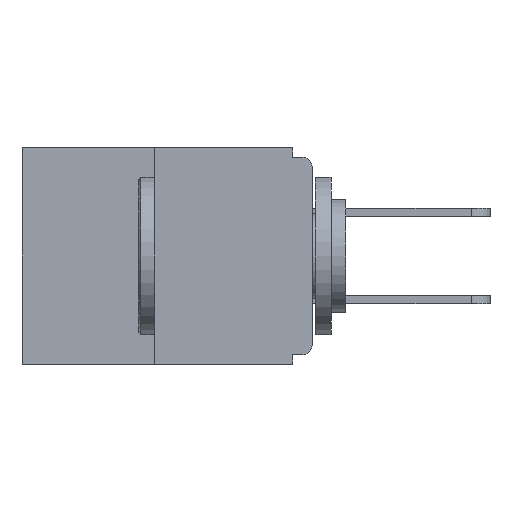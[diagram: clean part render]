
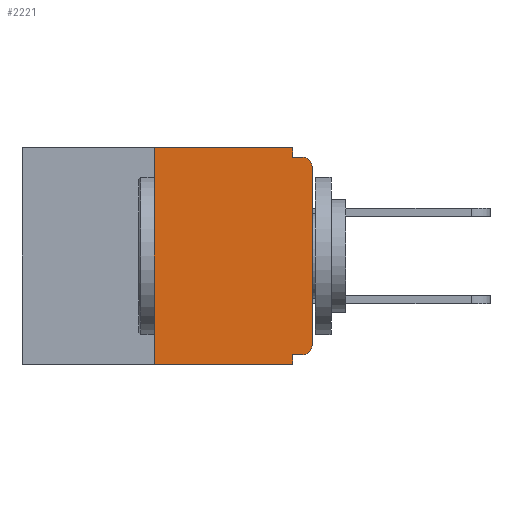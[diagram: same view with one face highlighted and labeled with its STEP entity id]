
A CAD part, left-side view. The second image highlights one B-rep face of the part: STEP entity #2221.
In plain terms, the highlighted planar face has unit normal (-1, 0, 0).
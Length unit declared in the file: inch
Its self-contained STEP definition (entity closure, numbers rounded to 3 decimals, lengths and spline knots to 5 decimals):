
#11 = CARTESIAN_POINT ( 'NONE',  ( 0., 0.031, -0.015 ) ) ;
#35 = DIRECTION ( 'NONE',  ( 1., 0., 0. ) ) ;
#146 = CARTESIAN_POINT ( 'NONE',  ( 0., 0., -0.328 ) ) ;
#283 = EDGE_CURVE ( 'NONE', #6004, #7386, #11529, .T. ) ;
#338 = CARTESIAN_POINT ( 'NONE',  ( 0., 0.031, 0. ) ) ;
#627 = AXIS2_PLACEMENT_3D ( 'NONE', #953, #35, #7451 ) ;
#688 = EDGE_CURVE ( 'NONE', #5996, #1993, #7983, .T. ) ;
#821 = DIRECTION ( 'NONE',  ( 0., 0., 1. ) ) ;
#953 = CARTESIAN_POINT ( 'NONE',  ( 0., 0.46, 0. ) ) ;
#961 = ORIENTED_EDGE ( 'NONE', *, *, #6815, .F. ) ;
#1276 = LINE ( 'NONE', #10023, #9420 ) ;
#1519 = VERTEX_POINT ( 'NONE', #7394 ) ;
#1734 = EDGE_CURVE ( 'NONE', #5830, #1993, #1919, .T. ) ;
#1814 = ORIENTED_EDGE ( 'NONE', *, *, #283, .F. ) ;
#1919 = LINE ( 'NONE', #5039, #4469 ) ;
#1963 = VERTEX_POINT ( 'NONE', #5065 ) ;
#1993 = VERTEX_POINT ( 'NONE', #6991 ) ;
#2065 = CARTESIAN_POINT ( 'NONE',  ( 0., 0., -0.03 ) ) ;
#2221 = ADVANCED_FACE ( 'NONE', ( #7251 ), #2738, .F. ) ;
#2358 = DIRECTION ( 'NONE',  ( 0., -1., 0. ) ) ;
#2637 = CARTESIAN_POINT ( 'NONE',  ( 0., 0.031, -0.343 ) ) ;
#2713 = VECTOR ( 'NONE', #10312, 39.37008 ) ;
#2722 = VERTEX_POINT ( 'NONE', #8371 ) ;
#2738 = PLANE ( 'NONE',  #627 ) ;
#2807 = DIRECTION ( 'NONE',  ( -1., 0., 0. ) ) ;
#2869 = DIRECTION ( 'NONE',  ( 0., 0., -1. ) ) ;
#2889 = CARTESIAN_POINT ( 'NONE',  ( 0., 0.25, 0. ) ) ;
#2900 = CARTESIAN_POINT ( 'NONE',  ( 0., 0.015, -0.03 ) ) ;
#3230 = EDGE_CURVE ( 'NONE', #7386, #5830, #5645, .T. ) ;
#3302 = EDGE_CURVE ( 'NONE', #11830, #5996, #1276, .T. ) ;
#3470 = LINE ( 'NONE', #2637, #6813 ) ;
#3475 = ORIENTED_EDGE ( 'NONE', *, *, #1734, .F. ) ;
#3624 = AXIS2_PLACEMENT_3D ( 'NONE', #4857, #5897, #11465 ) ;
#3935 = CARTESIAN_POINT ( 'NONE',  ( 0., 0.031, 0. ) ) ;
#4205 = DIRECTION ( 'NONE',  ( 0., -1., 0. ) ) ;
#4469 = VECTOR ( 'NONE', #2358, 39.37008 ) ;
#4768 = VECTOR ( 'NONE', #4800, 39.37008 ) ;
#4800 = DIRECTION ( 'NONE',  ( 0., 1., 0. ) ) ;
#4832 = EDGE_CURVE ( 'NONE', #1519, #6004, #6528, .T. ) ;
#4857 = CARTESIAN_POINT ( 'NONE',  ( 0., 0.015, -0.313 ) ) ;
#4876 = VECTOR ( 'NONE', #4205, 39.37008 ) ;
#5039 = CARTESIAN_POINT ( 'NONE',  ( 0., 0., -0.015 ) ) ;
#5065 = CARTESIAN_POINT ( 'NONE',  ( 0., 0.031, -0.328 ) ) ;
#5296 = AXIS2_PLACEMENT_3D ( 'NONE', #2900, #2807, #8554 ) ;
#5645 = LINE ( 'NONE', #3935, #7877 ) ;
#5830 = VERTEX_POINT ( 'NONE', #11 ) ;
#5897 = DIRECTION ( 'NONE',  ( -1., 0., 0. ) ) ;
#5996 = VERTEX_POINT ( 'NONE', #2065 ) ;
#6004 = VERTEX_POINT ( 'NONE', #2889 ) ;
#6528 = LINE ( 'NONE', #10092, #11297 ) ;
#6536 = LINE ( 'NONE', #146, #4768 ) ;
#6705 = CARTESIAN_POINT ( 'NONE',  ( 0., 0.015, -0.328 ) ) ;
#6813 = VECTOR ( 'NONE', #7331, 39.37008 ) ;
#6815 = EDGE_CURVE ( 'NONE', #7928, #1963, #6536, .T. ) ;
#6991 = CARTESIAN_POINT ( 'NONE',  ( 0., 0.015, -0.015 ) ) ;
#7065 = LINE ( 'NONE', #8900, #4876 ) ;
#7251 = FACE_OUTER_BOUND ( 'NONE', #8173, .T. ) ;
#7331 = DIRECTION ( 'NONE',  ( 0., 0., -1. ) ) ;
#7386 = VERTEX_POINT ( 'NONE', #338 ) ;
#7394 = CARTESIAN_POINT ( 'NONE',  ( 0., 0.25, -0.343 ) ) ;
#7451 = DIRECTION ( 'NONE',  ( 0., 0., -1. ) ) ;
#7676 = EDGE_CURVE ( 'NONE', #1963, #2722, #3470, .T. ) ;
#7817 = CARTESIAN_POINT ( 'NONE',  ( 0., 0., -0.313 ) ) ;
#7877 = VECTOR ( 'NONE', #2869, 39.37008 ) ;
#7902 = EDGE_CURVE ( 'NONE', #7928, #11830, #9017, .T. ) ;
#7928 = VERTEX_POINT ( 'NONE', #6705 ) ;
#7983 = CIRCLE ( 'NONE', #5296, 0.015 ) ;
#8099 = ORIENTED_EDGE ( 'NONE', *, *, #4832, .F. ) ;
#8133 = DIRECTION ( 'NONE',  ( 0., 0., 1. ) ) ;
#8173 = EDGE_LOOP ( 'NONE', ( #1814, #8099, #8597, #11131, #961, #8685, #9790, #9834, #3475, #11648 ) ) ;
#8255 = EDGE_CURVE ( 'NONE', #1519, #2722, #7065, .T. ) ;
#8371 = CARTESIAN_POINT ( 'NONE',  ( 0., 0.031, -0.343 ) ) ;
#8554 = DIRECTION ( 'NONE',  ( 0., 0., -1. ) ) ;
#8597 = ORIENTED_EDGE ( 'NONE', *, *, #8255, .T. ) ;
#8685 = ORIENTED_EDGE ( 'NONE', *, *, #7902, .T. ) ;
#8900 = CARTESIAN_POINT ( 'NONE',  ( 0., 0.46, -0.343 ) ) ;
#9017 = CIRCLE ( 'NONE', #3624, 0.015 ) ;
#9401 = CARTESIAN_POINT ( 'NONE',  ( 0., 0.46, 0. ) ) ;
#9420 = VECTOR ( 'NONE', #821, 39.37008 ) ;
#9790 = ORIENTED_EDGE ( 'NONE', *, *, #3302, .T. ) ;
#9834 = ORIENTED_EDGE ( 'NONE', *, *, #688, .T. ) ;
#10023 = CARTESIAN_POINT ( 'NONE',  ( 0., 0., 0. ) ) ;
#10092 = CARTESIAN_POINT ( 'NONE',  ( 0., 0.25, 0. ) ) ;
#10312 = DIRECTION ( 'NONE',  ( 0., -1., 0. ) ) ;
#11131 = ORIENTED_EDGE ( 'NONE', *, *, #7676, .F. ) ;
#11297 = VECTOR ( 'NONE', #8133, 39.37008 ) ;
#11465 = DIRECTION ( 'NONE',  ( 0., 0., -1. ) ) ;
#11529 = LINE ( 'NONE', #9401, #2713 ) ;
#11648 = ORIENTED_EDGE ( 'NONE', *, *, #3230, .F. ) ;
#11830 = VERTEX_POINT ( 'NONE', #7817 ) ;
